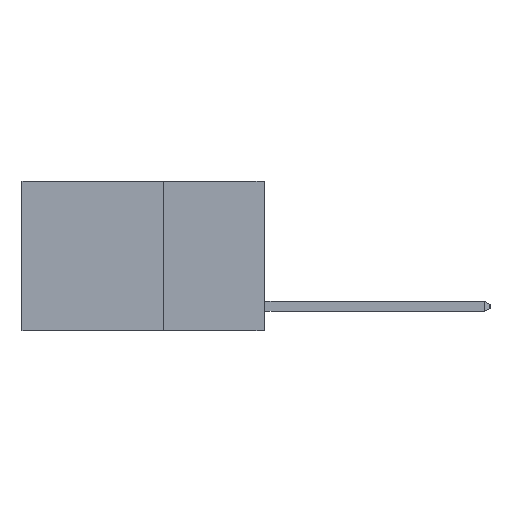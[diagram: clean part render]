
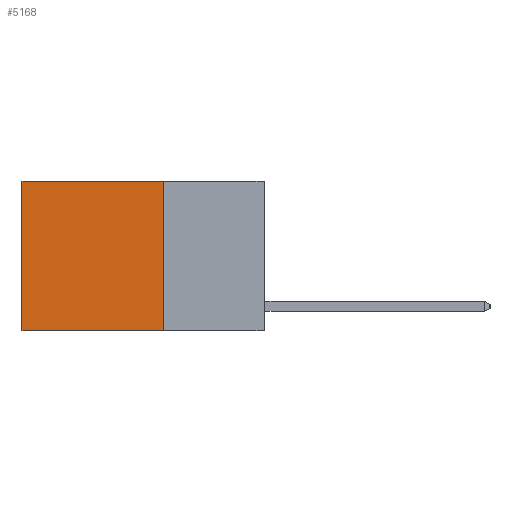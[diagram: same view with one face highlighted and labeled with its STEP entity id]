
A CAD part, left-side view. The second image highlights one B-rep face of the part: STEP entity #5168.
In plain terms, the highlighted planar face has unit normal (-1, 0, 0).
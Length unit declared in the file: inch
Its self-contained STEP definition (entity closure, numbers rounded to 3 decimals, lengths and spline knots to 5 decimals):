
#55 = ORIENTED_EDGE ( 'NONE', *, *, #15229, .F. ) ;
#1655 = LINE ( 'NONE', #3174, #14679 ) ;
#1931 = CARTESIAN_POINT ( 'NONE',  ( 0.2625, 0.6, -0.37 ) ) ;
#2246 = DIRECTION ( 'NONE',  ( 0., 1., 0. ) ) ;
#2341 = DIRECTION ( 'NONE',  ( 0., 0., -1. ) ) ;
#2903 = DIRECTION ( 'NONE',  ( 0., 0., -1. ) ) ;
#3174 = CARTESIAN_POINT ( 'NONE',  ( 0.2625, 0.25, -0.37 ) ) ;
#3642 = VERTEX_POINT ( 'NONE', #10061 ) ;
#4113 = VECTOR ( 'NONE', #2341, 39.37008 ) ;
#4527 = LINE ( 'NONE', #16111, #7854 ) ;
#5168 = ADVANCED_FACE ( 'NONE', ( #10930 ), #12963, .F. ) ;
#6940 = LINE ( 'NONE', #10471, #13269 ) ;
#7633 = EDGE_CURVE ( 'NONE', #13459, #9807, #4527, .T. ) ;
#7854 = VECTOR ( 'NONE', #2246, 39.37008 ) ;
#7920 = AXIS2_PLACEMENT_3D ( 'NONE', #10448, #14213, #2903 ) ;
#8247 = DIRECTION ( 'NONE',  ( 0., 1., 0. ) ) ;
#8249 = ORIENTED_EDGE ( 'NONE', *, *, #7633, .T. ) ;
#9633 = VERTEX_POINT ( 'NONE', #1931 ) ;
#9807 = VERTEX_POINT ( 'NONE', #13560 ) ;
#9884 = CARTESIAN_POINT ( 'NONE',  ( 0.2625, 0.25, 0. ) ) ;
#10026 = LINE ( 'NONE', #9884, #4113 ) ;
#10061 = CARTESIAN_POINT ( 'NONE',  ( 0.2625, 0.25, -0.37 ) ) ;
#10448 = CARTESIAN_POINT ( 'NONE',  ( 0.2625, 0.25, 0. ) ) ;
#10471 = CARTESIAN_POINT ( 'NONE',  ( 0.2625, 0.6, 0. ) ) ;
#10930 = FACE_OUTER_BOUND ( 'NONE', #11474, .T. ) ;
#11208 = CARTESIAN_POINT ( 'NONE',  ( 0.2625, 0.25, 0. ) ) ;
#11474 = EDGE_LOOP ( 'NONE', ( #12436, #12244, #55, #8249 ) ) ;
#11775 = DIRECTION ( 'NONE',  ( 0., 0., -1. ) ) ;
#12244 = ORIENTED_EDGE ( 'NONE', *, *, #12586, .F. ) ;
#12436 = ORIENTED_EDGE ( 'NONE', *, *, #13714, .T. ) ;
#12586 = EDGE_CURVE ( 'NONE', #3642, #9633, #1655, .T. ) ;
#12963 = PLANE ( 'NONE',  #7920 ) ;
#13269 = VECTOR ( 'NONE', #11775, 39.37008 ) ;
#13459 = VERTEX_POINT ( 'NONE', #11208 ) ;
#13560 = CARTESIAN_POINT ( 'NONE',  ( 0.2625, 0.6, 0. ) ) ;
#13714 = EDGE_CURVE ( 'NONE', #9807, #9633, #6940, .T. ) ;
#14213 = DIRECTION ( 'NONE',  ( 1., 0., 0. ) ) ;
#14679 = VECTOR ( 'NONE', #8247, 39.37008 ) ;
#15229 = EDGE_CURVE ( 'NONE', #13459, #3642, #10026, .T. ) ;
#16111 = CARTESIAN_POINT ( 'NONE',  ( 0.2625, 0.25, 0. ) ) ;
